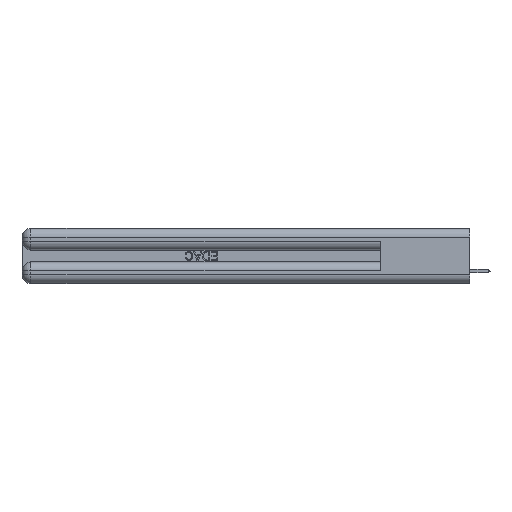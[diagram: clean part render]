
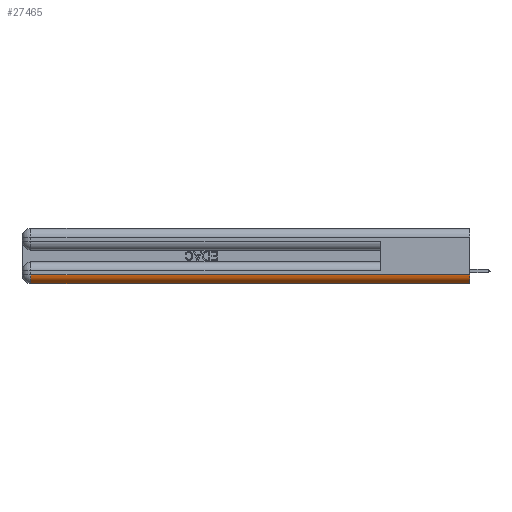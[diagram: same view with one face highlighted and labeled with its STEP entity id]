
A CAD part, left-side view. The second image highlights one B-rep face of the part: STEP entity #27465.
In plain terms, the highlighted cylindrical face has radius 1.524 mm (diameter 3.048 mm), a partial arc.
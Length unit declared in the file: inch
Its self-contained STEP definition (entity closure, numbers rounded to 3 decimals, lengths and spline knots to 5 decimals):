
#389 = CIRCLE ( 'NONE', #33353, 0.06 ) ;
#5044 = EDGE_CURVE ( 'NONE', #16545, #31506, #35766, .T. ) ;
#5202 = EDGE_LOOP ( 'NONE', ( #17651, #38224, #9201, #19803 ) ) ;
#6800 = CARTESIAN_POINT ( 'NONE',  ( 0.06, 0., 0.06 ) ) ;
#7624 = DIRECTION ( 'NONE',  ( 0., 1., 0. ) ) ;
#8008 = CARTESIAN_POINT ( 'NONE',  ( 0., 2.94, 0.06 ) ) ;
#9201 = ORIENTED_EDGE ( 'NONE', *, *, #19504, .F. ) ;
#10635 = CARTESIAN_POINT ( 'NONE',  ( 0., 0., 0.06 ) ) ;
#11507 = VECTOR ( 'NONE', #14031, 39.37008 ) ;
#13360 = VERTEX_POINT ( 'NONE', #28565 ) ;
#14031 = DIRECTION ( 'NONE',  ( 0., -1., 0. ) ) ;
#14904 = CIRCLE ( 'NONE', #22275, 0.06 ) ;
#16545 = VERTEX_POINT ( 'NONE', #18658 ) ;
#17043 = EDGE_CURVE ( 'NONE', #13360, #16545, #389, .T. ) ;
#17651 = ORIENTED_EDGE ( 'NONE', *, *, #17043, .F. ) ;
#18658 = CARTESIAN_POINT ( 'NONE',  ( 0.06, 0., 0. ) ) ;
#19504 = EDGE_CURVE ( 'NONE', #31506, #26125, #14904, .T. ) ;
#19791 = EDGE_CURVE ( 'NONE', #26125, #13360, #38457, .T. ) ;
#19803 = ORIENTED_EDGE ( 'NONE', *, *, #5044, .F. ) ;
#20435 = AXIS2_PLACEMENT_3D ( 'NONE', #6800, #28367, #37609 ) ;
#22275 = AXIS2_PLACEMENT_3D ( 'NONE', #26140, #7624, #29197 ) ;
#22615 = DIRECTION ( 'NONE',  ( 0., -1., 0. ) ) ;
#24276 = DIRECTION ( 'NONE',  ( 0., 1., 0. ) ) ;
#26125 = VERTEX_POINT ( 'NONE', #8008 ) ;
#26140 = CARTESIAN_POINT ( 'NONE',  ( 0.06, 2.94, 0.06 ) ) ;
#26617 = VECTOR ( 'NONE', #24276, 39.37008 ) ;
#27465 = ADVANCED_FACE ( 'NONE', ( #33937 ), #31493, .T. ) ;
#28367 = DIRECTION ( 'NONE',  ( 0., 1., 0. ) ) ;
#28565 = CARTESIAN_POINT ( 'NONE',  ( 0., 0., 0.06 ) ) ;
#28787 = DIRECTION ( 'NONE',  ( 0., 0., 1. ) ) ;
#29197 = DIRECTION ( 'NONE',  ( 0., 0., 1. ) ) ;
#31493 = CYLINDRICAL_SURFACE ( 'NONE', #20435, 0.06 ) ;
#31506 = VERTEX_POINT ( 'NONE', #38774 ) ;
#33353 = AXIS2_PLACEMENT_3D ( 'NONE', #37907, #22615, #28787 ) ;
#33562 = CARTESIAN_POINT ( 'NONE',  ( 0.06, 3., 0. ) ) ;
#33937 = FACE_OUTER_BOUND ( 'NONE', #5202, .T. ) ;
#35766 = LINE ( 'NONE', #33562, #26617 ) ;
#37609 = DIRECTION ( 'NONE',  ( 0., 0., 1. ) ) ;
#37907 = CARTESIAN_POINT ( 'NONE',  ( 0.06, 0., 0.06 ) ) ;
#38224 = ORIENTED_EDGE ( 'NONE', *, *, #19791, .F. ) ;
#38457 = LINE ( 'NONE', #10635, #11507 ) ;
#38774 = CARTESIAN_POINT ( 'NONE',  ( 0.06, 2.94, 0. ) ) ;
